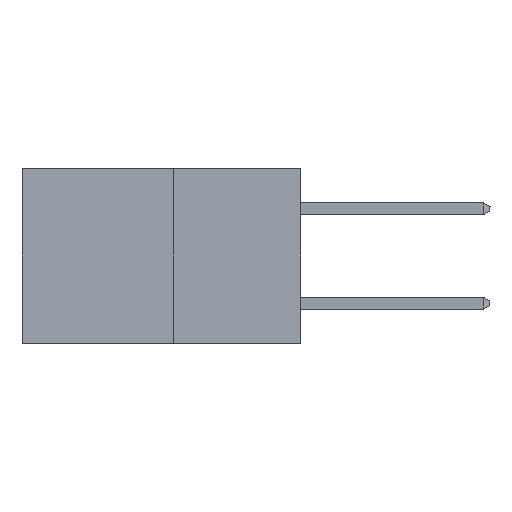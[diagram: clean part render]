
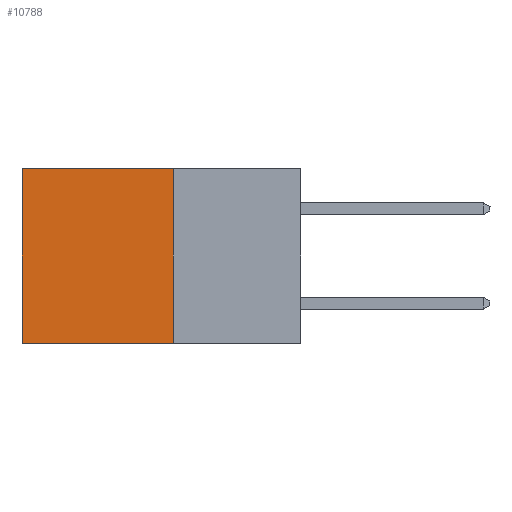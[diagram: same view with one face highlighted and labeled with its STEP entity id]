
A CAD part, left-side view. The second image highlights one B-rep face of the part: STEP entity #10788.
In plain terms, the highlighted planar face has unit normal (-1, 0, 0).
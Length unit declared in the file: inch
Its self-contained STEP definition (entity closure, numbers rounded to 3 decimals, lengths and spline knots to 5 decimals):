
#407 = DIRECTION ( 'NONE',  ( 0., 0., -1. ) ) ;
#424 = EDGE_LOOP ( 'NONE', ( #5018, #3567, #781, #8112 ) ) ;
#504 = LINE ( 'NONE', #10911, #9440 ) ;
#603 = CARTESIAN_POINT ( 'NONE',  ( 0.277, 0.27, -0.37 ) ) ;
#781 = ORIENTED_EDGE ( 'NONE', *, *, #1534, .F. ) ;
#926 = EDGE_CURVE ( 'NONE', #5976, #8792, #8081, .T. ) ;
#1144 = CARTESIAN_POINT ( 'NONE',  ( 0.277, 0.27, -0.37 ) ) ;
#1404 = LINE ( 'NONE', #6937, #8070 ) ;
#1534 = EDGE_CURVE ( 'NONE', #3753, #5976, #8277, .T. ) ;
#3567 = ORIENTED_EDGE ( 'NONE', *, *, #926, .F. ) ;
#3753 = VERTEX_POINT ( 'NONE', #7329 ) ;
#4413 = DIRECTION ( 'NONE',  ( 0., 0., -1. ) ) ;
#5018 = ORIENTED_EDGE ( 'NONE', *, *, #10436, .T. ) ;
#5246 = CARTESIAN_POINT ( 'NONE',  ( 0.277, 0.27, -0.37 ) ) ;
#5487 = VECTOR ( 'NONE', #7132, 39.37008 ) ;
#5673 = VERTEX_POINT ( 'NONE', #6318 ) ;
#5976 = VERTEX_POINT ( 'NONE', #1144 ) ;
#6228 = VECTOR ( 'NONE', #407, 39.37008 ) ;
#6318 = CARTESIAN_POINT ( 'NONE',  ( 0.277, 0.59, 0. ) ) ;
#6937 = CARTESIAN_POINT ( 'NONE',  ( 0.277, 0.27, 0. ) ) ;
#7086 = AXIS2_PLACEMENT_3D ( 'NONE', #5246, #9133, #4413 ) ;
#7132 = DIRECTION ( 'NONE',  ( 0., 1., 0. ) ) ;
#7329 = CARTESIAN_POINT ( 'NONE',  ( 0.277, 0.27, 0. ) ) ;
#7627 = PLANE ( 'NONE',  #7086 ) ;
#7741 = DIRECTION ( 'NONE',  ( 0., 1., 0. ) ) ;
#8051 = FACE_OUTER_BOUND ( 'NONE', #424, .T. ) ;
#8070 = VECTOR ( 'NONE', #7741, 39.37008 ) ;
#8081 = LINE ( 'NONE', #603, #5487 ) ;
#8112 = ORIENTED_EDGE ( 'NONE', *, *, #8522, .T. ) ;
#8164 = DIRECTION ( 'NONE',  ( 0., 0., -1. ) ) ;
#8277 = LINE ( 'NONE', #9900, #6228 ) ;
#8522 = EDGE_CURVE ( 'NONE', #3753, #5673, #1404, .T. ) ;
#8747 = CARTESIAN_POINT ( 'NONE',  ( 0.277, 0.59, -0.37 ) ) ;
#8792 = VERTEX_POINT ( 'NONE', #8747 ) ;
#9133 = DIRECTION ( 'NONE',  ( 1., 0., 0. ) ) ;
#9440 = VECTOR ( 'NONE', #8164, 39.37008 ) ;
#9900 = CARTESIAN_POINT ( 'NONE',  ( 0.277, 0.27, -0.37 ) ) ;
#10436 = EDGE_CURVE ( 'NONE', #5673, #8792, #504, .T. ) ;
#10788 = ADVANCED_FACE ( 'NONE', ( #8051 ), #7627, .F. ) ;
#10911 = CARTESIAN_POINT ( 'NONE',  ( 0.277, 0.59, -0.37 ) ) ;
